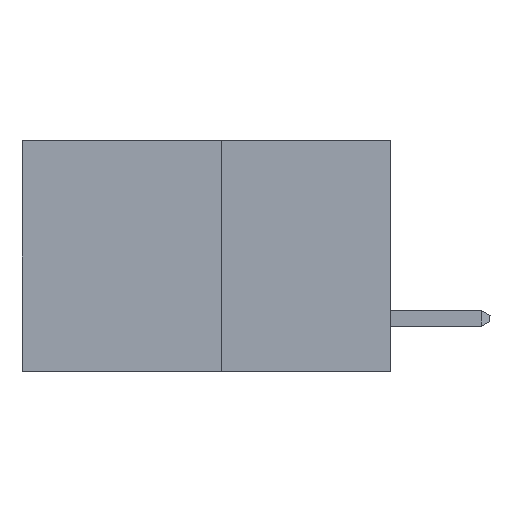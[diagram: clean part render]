
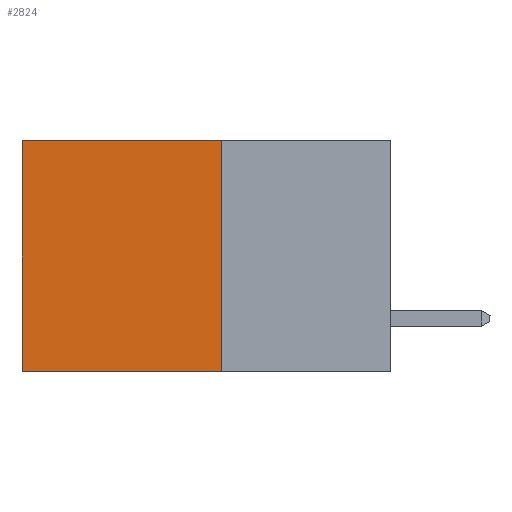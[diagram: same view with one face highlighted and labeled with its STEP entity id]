
A CAD part, left-side view. The second image highlights one B-rep face of the part: STEP entity #2824.
In plain terms, the highlighted planar face has unit normal (-1, 0, 0).
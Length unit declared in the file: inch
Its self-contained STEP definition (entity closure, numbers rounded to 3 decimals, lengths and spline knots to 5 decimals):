
#2 = VERTEX_POINT ( 'NONE', #11478 ) ;
#1296 = ORIENTED_EDGE ( 'NONE', *, *, #1852, .F. ) ;
#1852 = EDGE_CURVE ( 'NONE', #2, #11865, #12205, .T. ) ;
#2824 = ADVANCED_FACE ( 'NONE', ( #4132 ), #11095, .F. ) ;
#2921 = EDGE_CURVE ( 'NONE', #5146, #12886, #5540, .T. ) ;
#3083 = ORIENTED_EDGE ( 'NONE', *, *, #9563, .F. ) ;
#3562 = DIRECTION ( 'NONE',  ( 0., 1., 0. ) ) ;
#3616 = CARTESIAN_POINT ( 'NONE',  ( 0.277, 0.27, -0.37 ) ) ;
#4132 = FACE_OUTER_BOUND ( 'NONE', #8855, .T. ) ;
#4180 = AXIS2_PLACEMENT_3D ( 'NONE', #3616, #12247, #4938 ) ;
#4216 = VECTOR ( 'NONE', #9032, 39.37008 ) ;
#4938 = DIRECTION ( 'NONE',  ( 0., 0., -1. ) ) ;
#5146 = VERTEX_POINT ( 'NONE', #15747 ) ;
#5540 = LINE ( 'NONE', #10127, #15092 ) ;
#5750 = VECTOR ( 'NONE', #3562, 39.37008 ) ;
#6424 = LINE ( 'NONE', #16000, #4216 ) ;
#6561 = LINE ( 'NONE', #14222, #9508 ) ;
#8199 = EDGE_CURVE ( 'NONE', #12886, #11865, #6424, .T. ) ;
#8855 = EDGE_LOOP ( 'NONE', ( #12324, #1296, #3083, #10242 ) ) ;
#8918 = DIRECTION ( 'NONE',  ( 0., 1., 0. ) ) ;
#9032 = DIRECTION ( 'NONE',  ( 0., 0., -1. ) ) ;
#9508 = VECTOR ( 'NONE', #11949, 39.37008 ) ;
#9563 = EDGE_CURVE ( 'NONE', #5146, #2, #6561, .T. ) ;
#10127 = CARTESIAN_POINT ( 'NONE',  ( 0.277, 0.27, 0. ) ) ;
#10242 = ORIENTED_EDGE ( 'NONE', *, *, #2921, .T. ) ;
#11095 = PLANE ( 'NONE',  #4180 ) ;
#11478 = CARTESIAN_POINT ( 'NONE',  ( 0.277, 0.27, -0.37 ) ) ;
#11865 = VERTEX_POINT ( 'NONE', #12619 ) ;
#11949 = DIRECTION ( 'NONE',  ( 0., 0., -1. ) ) ;
#12054 = CARTESIAN_POINT ( 'NONE',  ( 0.277, 0.27, -0.37 ) ) ;
#12205 = LINE ( 'NONE', #12054, #5750 ) ;
#12247 = DIRECTION ( 'NONE',  ( 1., 0., 0. ) ) ;
#12324 = ORIENTED_EDGE ( 'NONE', *, *, #8199, .T. ) ;
#12619 = CARTESIAN_POINT ( 'NONE',  ( 0.277, 0.59, -0.37 ) ) ;
#12886 = VERTEX_POINT ( 'NONE', #14210 ) ;
#14210 = CARTESIAN_POINT ( 'NONE',  ( 0.277, 0.59, 0. ) ) ;
#14222 = CARTESIAN_POINT ( 'NONE',  ( 0.277, 0.27, -0.37 ) ) ;
#15092 = VECTOR ( 'NONE', #8918, 39.37008 ) ;
#15747 = CARTESIAN_POINT ( 'NONE',  ( 0.277, 0.27, 0. ) ) ;
#16000 = CARTESIAN_POINT ( 'NONE',  ( 0.277, 0.59, -0.37 ) ) ;
